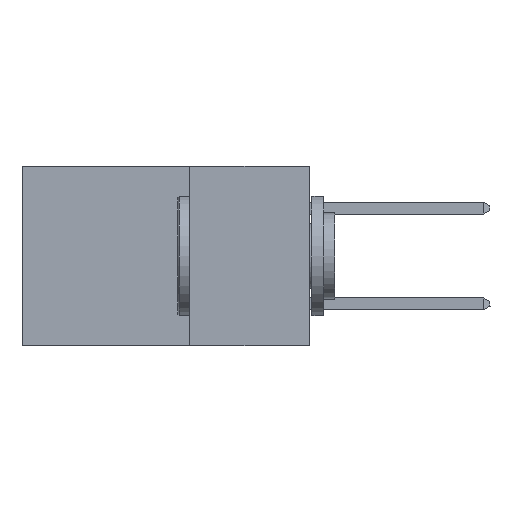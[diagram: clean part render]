
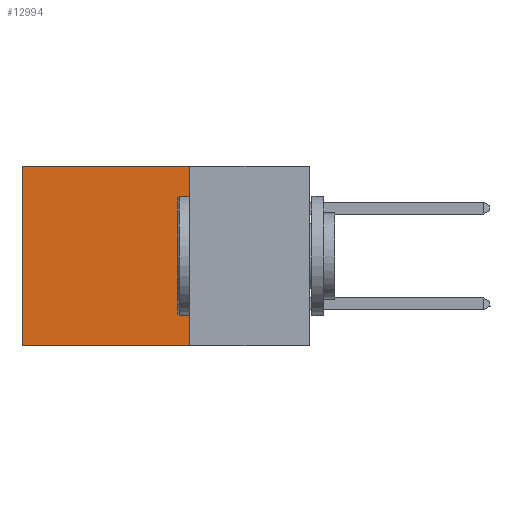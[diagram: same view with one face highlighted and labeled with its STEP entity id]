
A CAD part, left-side view. The second image highlights one B-rep face of the part: STEP entity #12994.
In plain terms, the highlighted planar face has unit normal (-1, 0, 0).
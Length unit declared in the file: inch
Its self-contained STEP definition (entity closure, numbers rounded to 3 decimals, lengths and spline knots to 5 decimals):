
#1256 = EDGE_CURVE ( 'NONE', #15018, #4002, #2152, .T. ) ;
#1652 = PLANE ( 'NONE',  #5131 ) ;
#2152 = LINE ( 'NONE', #9992, #2360 ) ;
#2360 = VECTOR ( 'NONE', #11531, 39.37008 ) ;
#2728 = CARTESIAN_POINT ( 'NONE',  ( 0.2875, 0.25, 0. ) ) ;
#3023 = EDGE_LOOP ( 'NONE', ( #16741, #10558, #10059, #5305 ) ) ;
#3304 = DIRECTION ( 'NONE',  ( 0., 0., -1. ) ) ;
#3694 = VECTOR ( 'NONE', #18153, 39.37008 ) ;
#4002 = VERTEX_POINT ( 'NONE', #8360 ) ;
#4352 = CARTESIAN_POINT ( 'NONE',  ( 0.2875, 0.6, -0.375 ) ) ;
#4992 = CARTESIAN_POINT ( 'NONE',  ( 0.2875, 0.25, 0. ) ) ;
#5131 = AXIS2_PLACEMENT_3D ( 'NONE', #6154, #10682, #3304 ) ;
#5305 = ORIENTED_EDGE ( 'NONE', *, *, #10548, .T. ) ;
#5615 = VERTEX_POINT ( 'NONE', #9980 ) ;
#6154 = CARTESIAN_POINT ( 'NONE',  ( 0.2875, 0.25, -0.375 ) ) ;
#6447 = DIRECTION ( 'NONE',  ( 0., 1., 0. ) ) ;
#6557 = LINE ( 'NONE', #4352, #16942 ) ;
#8360 = CARTESIAN_POINT ( 'NONE',  ( 0.2875, 0.6, -0.375 ) ) ;
#9980 = CARTESIAN_POINT ( 'NONE',  ( 0.2875, 0.6, 0. ) ) ;
#9992 = CARTESIAN_POINT ( 'NONE',  ( 0.2875, 0.25, -0.375 ) ) ;
#10059 = ORIENTED_EDGE ( 'NONE', *, *, #12492, .F. ) ;
#10548 = EDGE_CURVE ( 'NONE', #13416, #5615, #18771, .T. ) ;
#10558 = ORIENTED_EDGE ( 'NONE', *, *, #1256, .F. ) ;
#10682 = DIRECTION ( 'NONE',  ( 1., 0., 0. ) ) ;
#11157 = FACE_OUTER_BOUND ( 'NONE', #3023, .T. ) ;
#11531 = DIRECTION ( 'NONE',  ( 0., 1., 0. ) ) ;
#12248 = CARTESIAN_POINT ( 'NONE',  ( 0.2875, 0.25, -0.375 ) ) ;
#12492 = EDGE_CURVE ( 'NONE', #13416, #15018, #15698, .T. ) ;
#12994 = ADVANCED_FACE ( 'NONE', ( #11157 ), #1652, .F. ) ;
#13416 = VERTEX_POINT ( 'NONE', #2728 ) ;
#14686 = VECTOR ( 'NONE', #6447, 39.37008 ) ;
#14804 = DIRECTION ( 'NONE',  ( 0., 0., -1. ) ) ;
#15018 = VERTEX_POINT ( 'NONE', #19269 ) ;
#15698 = LINE ( 'NONE', #12248, #3694 ) ;
#16467 = EDGE_CURVE ( 'NONE', #5615, #4002, #6557, .T. ) ;
#16741 = ORIENTED_EDGE ( 'NONE', *, *, #16467, .T. ) ;
#16942 = VECTOR ( 'NONE', #14804, 39.37008 ) ;
#18153 = DIRECTION ( 'NONE',  ( 0., 0., -1. ) ) ;
#18771 = LINE ( 'NONE', #4992, #14686 ) ;
#19269 = CARTESIAN_POINT ( 'NONE',  ( 0.2875, 0.25, -0.375 ) ) ;
